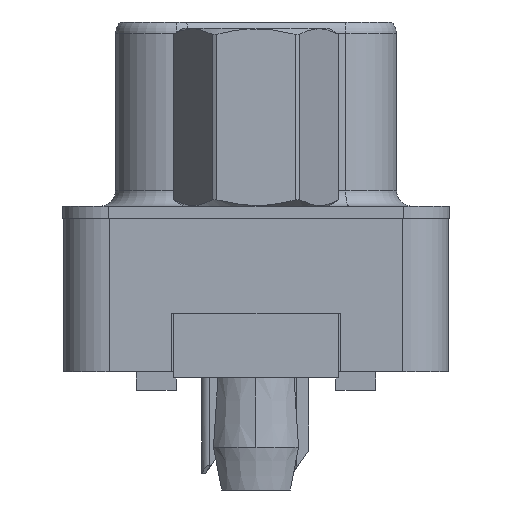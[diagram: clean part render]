
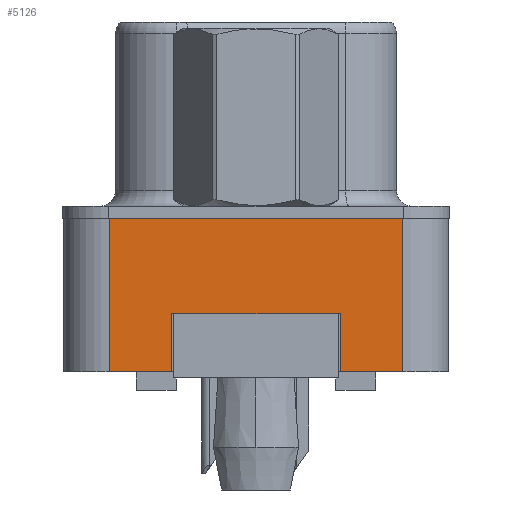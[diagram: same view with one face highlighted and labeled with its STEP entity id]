
A CAD part, left-side view. The second image highlights one B-rep face of the part: STEP entity #5126.
In plain terms, the highlighted planar face has unit normal (-1, 0, 0).
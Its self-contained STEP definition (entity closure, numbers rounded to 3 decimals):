
#28 = VERTEX_POINT ( 'NONE', #9057 ) ;
#319 = CARTESIAN_POINT ( 'NONE',  ( -2.935, 4.775, -5. ) ) ;
#831 = LINE ( 'NONE', #14966, #6759 ) ;
#994 = DIRECTION ( 'NONE',  ( 0., -1., 0. ) ) ;
#1540 = DIRECTION ( 'NONE',  ( 0., 0., -1. ) ) ;
#2206 = VECTOR ( 'NONE', #6701, 1000. ) ;
#2247 = ORIENTED_EDGE ( 'NONE', *, *, #5603, .F. ) ;
#2397 = VERTEX_POINT ( 'NONE', #319 ) ;
#2520 = DIRECTION ( 'NONE',  ( 0., 0., -1. ) ) ;
#2999 = DIRECTION ( 'NONE',  ( 0., 0., 1. ) ) ;
#3166 = LINE ( 'NONE', #3818, #8702 ) ;
#3332 = EDGE_CURVE ( 'NONE', #4332, #5401, #13267, .T. ) ;
#3366 = VERTEX_POINT ( 'NONE', #20235 ) ;
#3818 = CARTESIAN_POINT ( 'NONE',  ( -2.935, -2.75, -3.1 ) ) ;
#3998 = EDGE_CURVE ( 'NONE', #2397, #21097, #17360, .T. ) ;
#4044 = VERTEX_POINT ( 'NONE', #22932 ) ;
#4332 = VERTEX_POINT ( 'NONE', #9586 ) ;
#4474 = DIRECTION ( 'NONE',  ( 0., -1., 0. ) ) ;
#5058 = FACE_OUTER_BOUND ( 'NONE', #12770, .T. ) ;
#5126 = ADVANCED_FACE ( 'NONE', ( #5058 ), #6378, .T. ) ;
#5401 = VERTEX_POINT ( 'NONE', #21266 ) ;
#5603 = EDGE_CURVE ( 'NONE', #28, #3366, #21838, .T. ) ;
#6218 = CARTESIAN_POINT ( 'NONE',  ( -2.935, -4.775, -5. ) ) ;
#6228 = ORIENTED_EDGE ( 'NONE', *, *, #3998, .T. ) ;
#6378 = PLANE ( 'NONE',  #10589 ) ;
#6482 = LINE ( 'NONE', #13557, #22078 ) ;
#6701 = DIRECTION ( 'NONE',  ( 0., -1., 0. ) ) ;
#6759 = VECTOR ( 'NONE', #8342, 1000. ) ;
#7286 = VERTEX_POINT ( 'NONE', #9299 ) ;
#7397 = VECTOR ( 'NONE', #11040, 1000. ) ;
#7633 = EDGE_CURVE ( 'NONE', #3366, #21097, #18289, .T. ) ;
#8046 = CARTESIAN_POINT ( 'NONE',  ( -2.935, -4.775, 0. ) ) ;
#8342 = DIRECTION ( 'NONE',  ( 0., 0., 1. ) ) ;
#8702 = VECTOR ( 'NONE', #1540, 1000. ) ;
#9057 = CARTESIAN_POINT ( 'NONE',  ( -2.935, -2.75, -3.1 ) ) ;
#9194 = ORIENTED_EDGE ( 'NONE', *, *, #11327, .T. ) ;
#9299 = CARTESIAN_POINT ( 'NONE',  ( -2.935, -4.775, -5. ) ) ;
#9586 = CARTESIAN_POINT ( 'NONE',  ( -2.935, 4.775, 0. ) ) ;
#9967 = DIRECTION ( 'NONE',  ( -1., 0., 0. ) ) ;
#10589 = AXIS2_PLACEMENT_3D ( 'NONE', #15604, #9967, #20536 ) ;
#10732 = EDGE_CURVE ( 'NONE', #4044, #7286, #17113, .T. ) ;
#11040 = DIRECTION ( 'NONE',  ( 0., 1., 0. ) ) ;
#11327 = EDGE_CURVE ( 'NONE', #28, #4044, #3166, .T. ) ;
#11697 = EDGE_CURVE ( 'NONE', #7286, #5401, #6482, .T. ) ;
#12476 = ORIENTED_EDGE ( 'NONE', *, *, #3332, .F. ) ;
#12770 = EDGE_LOOP ( 'NONE', ( #9194, #17958, #22172, #12476, #19727, #6228, #15478, #2247 ) ) ;
#13267 = LINE ( 'NONE', #8046, #18586 ) ;
#13557 = CARTESIAN_POINT ( 'NONE',  ( -2.935, -4.775, -5. ) ) ;
#14966 = CARTESIAN_POINT ( 'NONE',  ( -2.935, 4.775, -5. ) ) ;
#15165 = CARTESIAN_POINT ( 'NONE',  ( -2.935, 2.75, -5. ) ) ;
#15478 = ORIENTED_EDGE ( 'NONE', *, *, #7633, .F. ) ;
#15604 = CARTESIAN_POINT ( 'NONE',  ( -2.935, -4.775, -5. ) ) ;
#15968 = CARTESIAN_POINT ( 'NONE',  ( -2.935, -4.775, -5. ) ) ;
#17113 = LINE ( 'NONE', #6218, #19494 ) ;
#17360 = LINE ( 'NONE', #15968, #2206 ) ;
#17958 = ORIENTED_EDGE ( 'NONE', *, *, #10732, .T. ) ;
#18006 = CARTESIAN_POINT ( 'NONE',  ( -2.935, 2.75, -3.1 ) ) ;
#18055 = EDGE_CURVE ( 'NONE', #2397, #4332, #831, .T. ) ;
#18289 = LINE ( 'NONE', #18409, #21101 ) ;
#18409 = CARTESIAN_POINT ( 'NONE',  ( -2.935, 2.75, -3.1 ) ) ;
#18586 = VECTOR ( 'NONE', #994, 1000. ) ;
#19494 = VECTOR ( 'NONE', #4474, 1000. ) ;
#19727 = ORIENTED_EDGE ( 'NONE', *, *, #18055, .F. ) ;
#20235 = CARTESIAN_POINT ( 'NONE',  ( -2.935, 2.75, -3.1 ) ) ;
#20536 = DIRECTION ( 'NONE',  ( 0., 0., 1. ) ) ;
#21097 = VERTEX_POINT ( 'NONE', #15165 ) ;
#21101 = VECTOR ( 'NONE', #2520, 1000. ) ;
#21266 = CARTESIAN_POINT ( 'NONE',  ( -2.935, -4.775, 0. ) ) ;
#21838 = LINE ( 'NONE', #18006, #7397 ) ;
#22078 = VECTOR ( 'NONE', #2999, 1000. ) ;
#22172 = ORIENTED_EDGE ( 'NONE', *, *, #11697, .T. ) ;
#22932 = CARTESIAN_POINT ( 'NONE',  ( -2.935, -2.75, -5. ) ) ;
